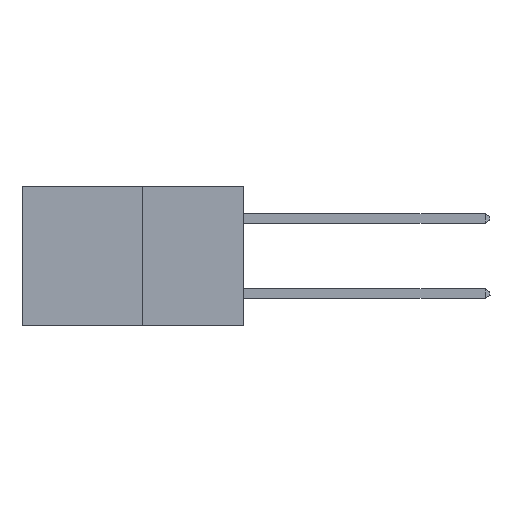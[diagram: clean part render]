
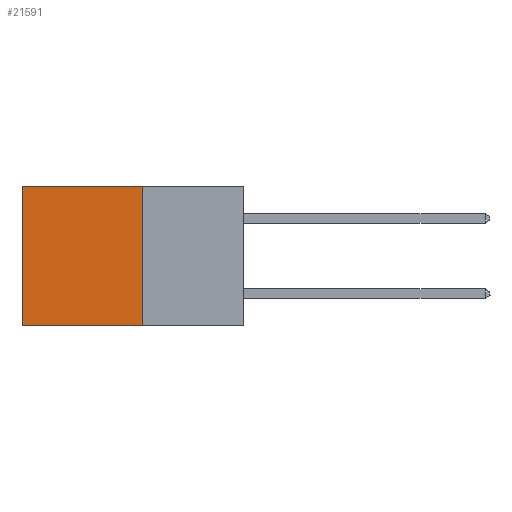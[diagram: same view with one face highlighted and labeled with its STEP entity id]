
A CAD part, left-side view. The second image highlights one B-rep face of the part: STEP entity #21591.
In plain terms, the highlighted planar face has unit normal (-1, 0, 0).
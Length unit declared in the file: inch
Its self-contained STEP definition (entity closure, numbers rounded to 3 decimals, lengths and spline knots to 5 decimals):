
#909 = EDGE_LOOP ( 'NONE', ( #9920, #12030, #1902, #3021 ) ) ;
#1369 = FACE_OUTER_BOUND ( 'NONE', #909, .T. ) ;
#1902 = ORIENTED_EDGE ( 'NONE', *, *, #17572, .F. ) ;
#2773 = LINE ( 'NONE', #13580, #25455 ) ;
#3021 = ORIENTED_EDGE ( 'NONE', *, *, #9254, .T. ) ;
#3075 = CARTESIAN_POINT ( 'NONE',  ( 0.277, 0.27, 0. ) ) ;
#3390 = EDGE_CURVE ( 'NONE', #5208, #9696, #2773, .T. ) ;
#3985 = CARTESIAN_POINT ( 'NONE',  ( 0.277, 0.59, 0. ) ) ;
#5170 = DIRECTION ( 'NONE',  ( 1., 0., 0. ) ) ;
#5208 = VERTEX_POINT ( 'NONE', #14568 ) ;
#7369 = CARTESIAN_POINT ( 'NONE',  ( 0.277, 0.59, -0.37 ) ) ;
#9254 = EDGE_CURVE ( 'NONE', #25805, #20502, #22656, .T. ) ;
#9354 = PLANE ( 'NONE',  #18034 ) ;
#9696 = VERTEX_POINT ( 'NONE', #7369 ) ;
#9920 = ORIENTED_EDGE ( 'NONE', *, *, #27145, .T. ) ;
#9950 = VECTOR ( 'NONE', #14467, 39.37008 ) ;
#12030 = ORIENTED_EDGE ( 'NONE', *, *, #3390, .F. ) ;
#13555 = DIRECTION ( 'NONE',  ( 0., 1., 0. ) ) ;
#13580 = CARTESIAN_POINT ( 'NONE',  ( 0.277, 0.27, -0.37 ) ) ;
#13611 = CARTESIAN_POINT ( 'NONE',  ( 0.277, 0.27, -0.37 ) ) ;
#14467 = DIRECTION ( 'NONE',  ( 0., 1., 0. ) ) ;
#14568 = CARTESIAN_POINT ( 'NONE',  ( 0.277, 0.27, -0.37 ) ) ;
#15369 = VECTOR ( 'NONE', #20180, 39.37008 ) ;
#16195 = VECTOR ( 'NONE', #20605, 39.37008 ) ;
#16855 = LINE ( 'NONE', #18450, #16195 ) ;
#17572 = EDGE_CURVE ( 'NONE', #25805, #5208, #27296, .T. ) ;
#17970 = CARTESIAN_POINT ( 'NONE',  ( 0.277, 0.27, -0.37 ) ) ;
#18034 = AXIS2_PLACEMENT_3D ( 'NONE', #17970, #5170, #20115 ) ;
#18450 = CARTESIAN_POINT ( 'NONE',  ( 0.277, 0.59, -0.37 ) ) ;
#18774 = CARTESIAN_POINT ( 'NONE',  ( 0.277, 0.27, 0. ) ) ;
#20115 = DIRECTION ( 'NONE',  ( 0., 0., -1. ) ) ;
#20180 = DIRECTION ( 'NONE',  ( 0., 0., -1. ) ) ;
#20502 = VERTEX_POINT ( 'NONE', #3985 ) ;
#20605 = DIRECTION ( 'NONE',  ( 0., 0., -1. ) ) ;
#21591 = ADVANCED_FACE ( 'NONE', ( #1369 ), #9354, .F. ) ;
#22656 = LINE ( 'NONE', #18774, #9950 ) ;
#25455 = VECTOR ( 'NONE', #13555, 39.37008 ) ;
#25805 = VERTEX_POINT ( 'NONE', #3075 ) ;
#27145 = EDGE_CURVE ( 'NONE', #20502, #9696, #16855, .T. ) ;
#27296 = LINE ( 'NONE', #13611, #15369 ) ;
